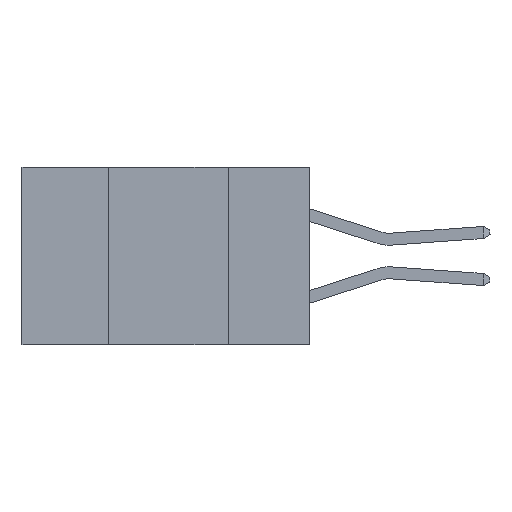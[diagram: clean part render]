
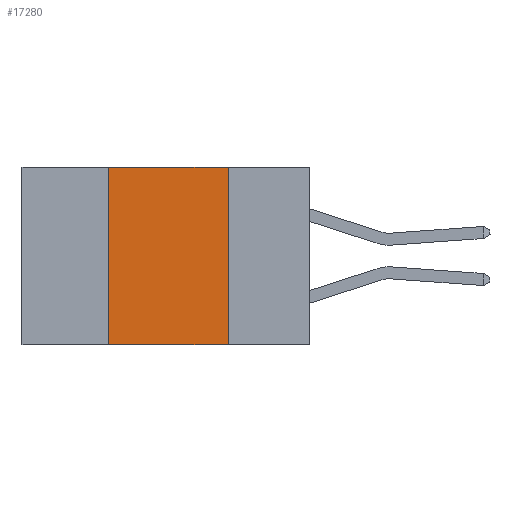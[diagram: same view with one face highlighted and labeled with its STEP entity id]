
A CAD part, left-side view. The second image highlights one B-rep face of the part: STEP entity #17280.
In plain terms, the highlighted planar face has unit normal (-1, 0, 0).
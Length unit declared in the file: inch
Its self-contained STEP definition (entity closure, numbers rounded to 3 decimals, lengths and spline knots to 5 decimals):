
#418 = EDGE_CURVE ( 'NONE', #19691, #16149, #1156, .T. ) ;
#1088 = VECTOR ( 'NONE', #11011, 39.37008 ) ;
#1156 = LINE ( 'NONE', #20914, #2918 ) ;
#1601 = CARTESIAN_POINT ( 'NONE',  ( 0., 0.42, 0. ) ) ;
#1676 = CARTESIAN_POINT ( 'NONE',  ( 0., 0.17, 0. ) ) ;
#2918 = VECTOR ( 'NONE', #7773, 39.37008 ) ;
#4418 = AXIS2_PLACEMENT_3D ( 'NONE', #5346, #8547, #15185 ) ;
#4433 = ORIENTED_EDGE ( 'NONE', *, *, #418, .F. ) ;
#5346 = CARTESIAN_POINT ( 'NONE',  ( 0., 0.6, 0. ) ) ;
#7519 = VERTEX_POINT ( 'NONE', #9235 ) ;
#7773 = DIRECTION ( 'NONE',  ( 0., 0., -1. ) ) ;
#8371 = LINE ( 'NONE', #14887, #11311 ) ;
#8475 = DIRECTION ( 'NONE',  ( 0., -1., 0. ) ) ;
#8547 = DIRECTION ( 'NONE',  ( 1., 0., 0. ) ) ;
#8815 = LINE ( 'NONE', #13727, #9371 ) ;
#9172 = EDGE_CURVE ( 'NONE', #11475, #19691, #8371, .T. ) ;
#9235 = CARTESIAN_POINT ( 'NONE',  ( 0., 0.42, -0.37 ) ) ;
#9274 = CARTESIAN_POINT ( 'NONE',  ( 0., 0.17, -0.37 ) ) ;
#9371 = VECTOR ( 'NONE', #15442, 39.37008 ) ;
#11011 = DIRECTION ( 'NONE',  ( 0., 0., 1. ) ) ;
#11106 = LINE ( 'NONE', #15839, #1088 ) ;
#11311 = VECTOR ( 'NONE', #8475, 39.37008 ) ;
#11475 = VERTEX_POINT ( 'NONE', #1601 ) ;
#11562 = ORIENTED_EDGE ( 'NONE', *, *, #13661, .F. ) ;
#11635 = PLANE ( 'NONE',  #4418 ) ;
#12194 = ORIENTED_EDGE ( 'NONE', *, *, #20736, .T. ) ;
#13661 = EDGE_CURVE ( 'NONE', #7519, #11475, #11106, .T. ) ;
#13669 = FACE_OUTER_BOUND ( 'NONE', #17706, .T. ) ;
#13727 = CARTESIAN_POINT ( 'NONE',  ( 0., 0.6, -0.37 ) ) ;
#14887 = CARTESIAN_POINT ( 'NONE',  ( 0., 0.6, 0. ) ) ;
#15185 = DIRECTION ( 'NONE',  ( 0., 0., -1. ) ) ;
#15442 = DIRECTION ( 'NONE',  ( 0., -1., 0. ) ) ;
#15839 = CARTESIAN_POINT ( 'NONE',  ( 0., 0.42, -0.37 ) ) ;
#16149 = VERTEX_POINT ( 'NONE', #9274 ) ;
#17280 = ADVANCED_FACE ( 'NONE', ( #13669 ), #11635, .F. ) ;
#17706 = EDGE_LOOP ( 'NONE', ( #4433, #18609, #11562, #12194 ) ) ;
#18609 = ORIENTED_EDGE ( 'NONE', *, *, #9172, .F. ) ;
#19691 = VERTEX_POINT ( 'NONE', #1676 ) ;
#20736 = EDGE_CURVE ( 'NONE', #7519, #16149, #8815, .T. ) ;
#20914 = CARTESIAN_POINT ( 'NONE',  ( 0., 0.17, -0.37 ) ) ;
